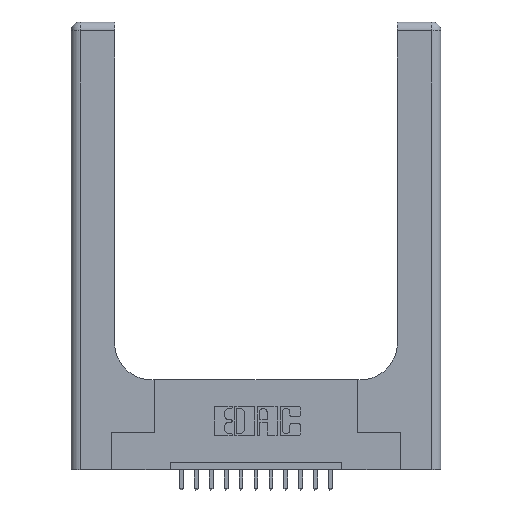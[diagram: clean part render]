
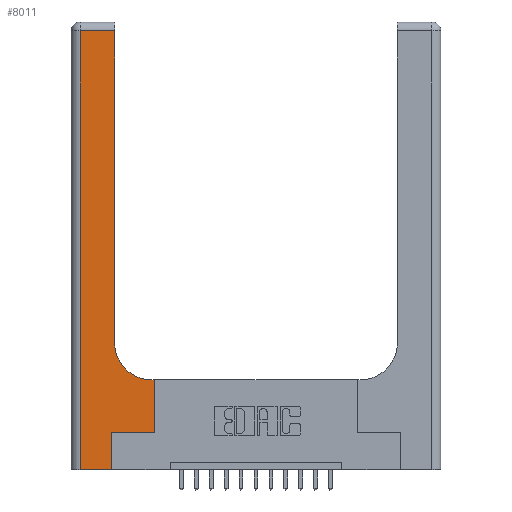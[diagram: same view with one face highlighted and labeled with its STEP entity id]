
A CAD part, top view. The second image highlights one B-rep face of the part: STEP entity #8011.
In plain terms, the highlighted planar face has unit normal (0, 0, 1).
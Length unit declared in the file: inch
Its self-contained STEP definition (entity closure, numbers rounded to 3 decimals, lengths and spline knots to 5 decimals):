
#248 = CARTESIAN_POINT ( 'NONE',  ( 0.2915, 0.6, 0.37 ) ) ;
#422 = VECTOR ( 'NONE', #1906, 39.37008 ) ;
#650 = CARTESIAN_POINT ( 'NONE',  ( 0., 2.94, 0.37 ) ) ;
#749 = ORIENTED_EDGE ( 'NONE', *, *, #6481, .T. ) ;
#832 = LINE ( 'NONE', #1793, #14918 ) ;
#929 = LINE ( 'NONE', #16014, #16307 ) ;
#1063 = VERTEX_POINT ( 'NONE', #7402 ) ;
#1610 = CARTESIAN_POINT ( 'NONE',  ( 0.5415, 0.6, 0.37 ) ) ;
#1793 = CARTESIAN_POINT ( 'NONE',  ( 0., 0., 0.37 ) ) ;
#1906 = DIRECTION ( 'NONE',  ( -1., 0., 0. ) ) ;
#2034 = VECTOR ( 'NONE', #3304, 39.37008 ) ;
#2435 = VERTEX_POINT ( 'NONE', #4815 ) ;
#2551 = FACE_OUTER_BOUND ( 'NONE', #13011, .T. ) ;
#2638 = EDGE_CURVE ( 'NONE', #6306, #15573, #8679, .T. ) ;
#2748 = DIRECTION ( 'NONE',  ( 1., 0., 0. ) ) ;
#3274 = ORIENTED_EDGE ( 'NONE', *, *, #6099, .T. ) ;
#3304 = DIRECTION ( 'NONE',  ( -1., 0., 0. ) ) ;
#4098 = LINE ( 'NONE', #6434, #5189 ) ;
#4133 = PLANE ( 'NONE',  #14420 ) ;
#4586 = CARTESIAN_POINT ( 'NONE',  ( 0.269, 0., 0.37 ) ) ;
#4815 = CARTESIAN_POINT ( 'NONE',  ( 0.2915, 0.85, 0.37 ) ) ;
#5189 = VECTOR ( 'NONE', #15939, 39.37008 ) ;
#5286 = ORIENTED_EDGE ( 'NONE', *, *, #2638, .T. ) ;
#5339 = CARTESIAN_POINT ( 'NONE',  ( 0.06, 2.94, 0.37 ) ) ;
#6099 = EDGE_CURVE ( 'NONE', #12094, #10185, #15765, .T. ) ;
#6258 = CARTESIAN_POINT ( 'NONE',  ( 0.5585, 0.25, 0.37 ) ) ;
#6306 = VERTEX_POINT ( 'NONE', #9881 ) ;
#6434 = CARTESIAN_POINT ( 'NONE',  ( 0.269, 0., 0.37 ) ) ;
#6481 = EDGE_CURVE ( 'NONE', #10185, #10378, #14057, .T. ) ;
#6569 = DIRECTION ( 'NONE',  ( 0., -1., 0. ) ) ;
#6766 = DIRECTION ( 'NONE',  ( -1., 0., 0. ) ) ;
#7278 = ORIENTED_EDGE ( 'NONE', *, *, #14246, .T. ) ;
#7402 = CARTESIAN_POINT ( 'NONE',  ( 0.269, 0.25, 0.37 ) ) ;
#7647 = AXIS2_PLACEMENT_3D ( 'NONE', #17579, #7803, #2748 ) ;
#7803 = DIRECTION ( 'NONE',  ( 0., 0., -1. ) ) ;
#7816 = VECTOR ( 'NONE', #8614, 39.37008 ) ;
#8011 = ADVANCED_FACE ( 'NONE', ( #2551 ), #4133, .F. ) ;
#8614 = DIRECTION ( 'NONE',  ( 1., 0., 0. ) ) ;
#8679 = LINE ( 'NONE', #248, #2034 ) ;
#8814 = EDGE_CURVE ( 'NONE', #15053, #1063, #4098, .T. ) ;
#9284 = DIRECTION ( 'NONE',  ( 0., 1., 0. ) ) ;
#9420 = DIRECTION ( 'NONE',  ( 0., 0., -1. ) ) ;
#9678 = ORIENTED_EDGE ( 'NONE', *, *, #17249, .T. ) ;
#9775 = ORIENTED_EDGE ( 'NONE', *, *, #14641, .T. ) ;
#9881 = CARTESIAN_POINT ( 'NONE',  ( 0.5585, 0.6, 0.37 ) ) ;
#10022 = DIRECTION ( 'NONE',  ( 1., 0., 0. ) ) ;
#10123 = LINE ( 'NONE', #10804, #11613 ) ;
#10185 = VERTEX_POINT ( 'NONE', #5339 ) ;
#10378 = VERTEX_POINT ( 'NONE', #13596 ) ;
#10804 = CARTESIAN_POINT ( 'NONE',  ( 0.2915, 3., 0.37 ) ) ;
#10987 = ORIENTED_EDGE ( 'NONE', *, *, #11429, .T. ) ;
#11429 = EDGE_CURVE ( 'NONE', #15573, #2435, #12796, .T. ) ;
#11613 = VECTOR ( 'NONE', #12173, 39.37008 ) ;
#11958 = EDGE_CURVE ( 'NONE', #10378, #15053, #832, .T. ) ;
#11976 = VERTEX_POINT ( 'NONE', #6258 ) ;
#12094 = VERTEX_POINT ( 'NONE', #14098 ) ;
#12173 = DIRECTION ( 'NONE',  ( 0., 1., 0. ) ) ;
#12468 = CARTESIAN_POINT ( 'NONE',  ( 0.269, 0.25, 0.37 ) ) ;
#12518 = ORIENTED_EDGE ( 'NONE', *, *, #11958, .T. ) ;
#12796 = CIRCLE ( 'NONE', #7647, 0.25 ) ;
#13011 = EDGE_LOOP ( 'NONE', ( #9775, #3274, #749, #12518, #16987, #7278, #9678, #5286, #10987 ) ) ;
#13596 = CARTESIAN_POINT ( 'NONE',  ( 0.06, 0., 0.37 ) ) ;
#14057 = LINE ( 'NONE', #14692, #16842 ) ;
#14098 = CARTESIAN_POINT ( 'NONE',  ( 0.2915, 2.94, 0.37 ) ) ;
#14246 = EDGE_CURVE ( 'NONE', #1063, #11976, #14385, .T. ) ;
#14385 = LINE ( 'NONE', #12468, #7816 ) ;
#14420 = AXIS2_PLACEMENT_3D ( 'NONE', #16513, #9420, #6766 ) ;
#14641 = EDGE_CURVE ( 'NONE', #2435, #12094, #10123, .T. ) ;
#14692 = CARTESIAN_POINT ( 'NONE',  ( 0.06, 3., 0.37 ) ) ;
#14918 = VECTOR ( 'NONE', #10022, 39.37008 ) ;
#15053 = VERTEX_POINT ( 'NONE', #4586 ) ;
#15573 = VERTEX_POINT ( 'NONE', #1610 ) ;
#15765 = LINE ( 'NONE', #650, #422 ) ;
#15939 = DIRECTION ( 'NONE',  ( 0., 1., 0. ) ) ;
#16014 = CARTESIAN_POINT ( 'NONE',  ( 0.5585, 0.25, 0.37 ) ) ;
#16307 = VECTOR ( 'NONE', #9284, 39.37008 ) ;
#16513 = CARTESIAN_POINT ( 'NONE',  ( 0., 3., 0.37 ) ) ;
#16842 = VECTOR ( 'NONE', #6569, 39.37008 ) ;
#16987 = ORIENTED_EDGE ( 'NONE', *, *, #8814, .T. ) ;
#17249 = EDGE_CURVE ( 'NONE', #11976, #6306, #929, .T. ) ;
#17579 = CARTESIAN_POINT ( 'NONE',  ( 0.5415, 0.85, 0.37 ) ) ;
